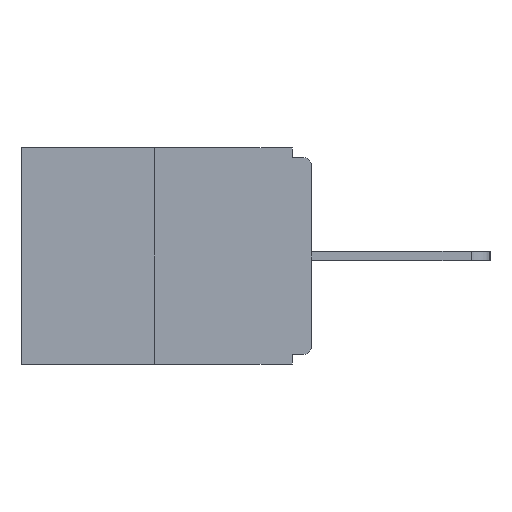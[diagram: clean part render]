
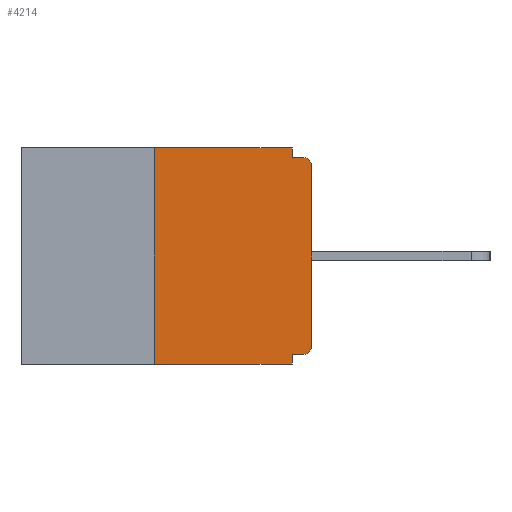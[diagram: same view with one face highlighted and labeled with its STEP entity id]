
A CAD part, left-side view. The second image highlights one B-rep face of the part: STEP entity #4214.
In plain terms, the highlighted planar face has unit normal (-1, 0, 0).
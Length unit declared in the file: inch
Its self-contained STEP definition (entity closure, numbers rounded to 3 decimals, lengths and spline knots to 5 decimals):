
#323 = AXIS2_PLACEMENT_3D ( 'NONE', #721, #25319, #17155 ) ;
#538 = ORIENTED_EDGE ( 'NONE', *, *, #24156, .F. ) ;
#721 = CARTESIAN_POINT ( 'NONE',  ( 0., 0.46, 0. ) ) ;
#915 = VECTOR ( 'NONE', #14910, 39.37008 ) ;
#925 = ORIENTED_EDGE ( 'NONE', *, *, #1506, .F. ) ;
#1203 = DIRECTION ( 'NONE',  ( 0., 0., -1. ) ) ;
#1506 = EDGE_CURVE ( 'NONE', #7267, #21298, #11425, .T. ) ;
#1704 = AXIS2_PLACEMENT_3D ( 'NONE', #9075, #2961, #7179 ) ;
#1990 = CARTESIAN_POINT ( 'NONE',  ( 0., 0.031, -0.015 ) ) ;
#2344 = EDGE_CURVE ( 'NONE', #15283, #7643, #25495, .T. ) ;
#2492 = FACE_OUTER_BOUND ( 'NONE', #23433, .T. ) ;
#2899 = EDGE_CURVE ( 'NONE', #25150, #3017, #26515, .T. ) ;
#2961 = DIRECTION ( 'NONE',  ( -1., 0., 0. ) ) ;
#3017 = VERTEX_POINT ( 'NONE', #17044 ) ;
#3369 = ORIENTED_EDGE ( 'NONE', *, *, #12321, .T. ) ;
#4214 = ADVANCED_FACE ( 'NONE', ( #2492 ), #15115, .F. ) ;
#4600 = CARTESIAN_POINT ( 'NONE',  ( 0., 0.25, -0.343 ) ) ;
#4879 = ORIENTED_EDGE ( 'NONE', *, *, #2899, .F. ) ;
#5553 = ORIENTED_EDGE ( 'NONE', *, *, #2344, .T. ) ;
#6460 = CIRCLE ( 'NONE', #22078, 0.015 ) ;
#6619 = CARTESIAN_POINT ( 'NONE',  ( 0., 0., -0.015 ) ) ;
#6686 = VECTOR ( 'NONE', #24481, 39.37008 ) ;
#6695 = ORIENTED_EDGE ( 'NONE', *, *, #18225, .F. ) ;
#6821 = LINE ( 'NONE', #12928, #9926 ) ;
#7179 = DIRECTION ( 'NONE',  ( 0., 0., -1. ) ) ;
#7267 = VERTEX_POINT ( 'NONE', #20975 ) ;
#7643 = VERTEX_POINT ( 'NONE', #8574 ) ;
#8574 = CARTESIAN_POINT ( 'NONE',  ( 0., 0., -0.03 ) ) ;
#9075 = CARTESIAN_POINT ( 'NONE',  ( 0., 0.015, -0.03 ) ) ;
#9462 = CARTESIAN_POINT ( 'NONE',  ( 0., 0., 0. ) ) ;
#9488 = CARTESIAN_POINT ( 'NONE',  ( 0., 0.031, 0. ) ) ;
#9853 = VECTOR ( 'NONE', #26040, 39.37008 ) ;
#9926 = VECTOR ( 'NONE', #13343, 39.37008 ) ;
#10602 = VERTEX_POINT ( 'NONE', #1990 ) ;
#10863 = CARTESIAN_POINT ( 'NONE',  ( 0., 0., -0.313 ) ) ;
#11134 = LINE ( 'NONE', #20710, #16124 ) ;
#11425 = LINE ( 'NONE', #15916, #22614 ) ;
#11450 = EDGE_CURVE ( 'NONE', #25150, #21298, #6821, .T. ) ;
#11519 = CARTESIAN_POINT ( 'NONE',  ( 0., 0.015, -0.313 ) ) ;
#12146 = CARTESIAN_POINT ( 'NONE',  ( 0., 0.031, -0.343 ) ) ;
#12321 = EDGE_CURVE ( 'NONE', #7643, #13069, #25129, .T. ) ;
#12851 = CARTESIAN_POINT ( 'NONE',  ( 0., 0.015, -0.328 ) ) ;
#12928 = CARTESIAN_POINT ( 'NONE',  ( 0., 0.46, -0.343 ) ) ;
#13044 = VECTOR ( 'NONE', #1203, 39.37008 ) ;
#13069 = VERTEX_POINT ( 'NONE', #13161 ) ;
#13161 = CARTESIAN_POINT ( 'NONE',  ( 0., 0.015, -0.015 ) ) ;
#13243 = CARTESIAN_POINT ( 'NONE',  ( 0., 0., -0.328 ) ) ;
#13343 = DIRECTION ( 'NONE',  ( 0., -1., 0. ) ) ;
#14123 = DIRECTION ( 'NONE',  ( -1., 0., 0. ) ) ;
#14910 = DIRECTION ( 'NONE',  ( 0., -1., 0. ) ) ;
#15115 = PLANE ( 'NONE',  #323 ) ;
#15283 = VERTEX_POINT ( 'NONE', #10863 ) ;
#15684 = ORIENTED_EDGE ( 'NONE', *, *, #26019, .F. ) ;
#15788 = DIRECTION ( 'NONE',  ( 0., 0., -1. ) ) ;
#15916 = CARTESIAN_POINT ( 'NONE',  ( 0., 0.031, -0.343 ) ) ;
#16124 = VECTOR ( 'NONE', #24782, 39.37008 ) ;
#16198 = CARTESIAN_POINT ( 'NONE',  ( 0., 0.25, 0. ) ) ;
#17044 = CARTESIAN_POINT ( 'NONE',  ( 0., 0.25, 0. ) ) ;
#17155 = DIRECTION ( 'NONE',  ( 0., 0., -1. ) ) ;
#18225 = EDGE_CURVE ( 'NONE', #24071, #7267, #25875, .T. ) ;
#18526 = ORIENTED_EDGE ( 'NONE', *, *, #22008, .T. ) ;
#18573 = VERTEX_POINT ( 'NONE', #19194 ) ;
#19194 = CARTESIAN_POINT ( 'NONE',  ( 0., 0.031, 0. ) ) ;
#19361 = DIRECTION ( 'NONE',  ( 0., 1., 0. ) ) ;
#20710 = CARTESIAN_POINT ( 'NONE',  ( 0., 0.46, 0. ) ) ;
#20907 = VECTOR ( 'NONE', #19361, 39.37008 ) ;
#20975 = CARTESIAN_POINT ( 'NONE',  ( 0., 0.031, -0.328 ) ) ;
#21298 = VERTEX_POINT ( 'NONE', #12146 ) ;
#22008 = EDGE_CURVE ( 'NONE', #24071, #15283, #6460, .T. ) ;
#22078 = AXIS2_PLACEMENT_3D ( 'NONE', #11519, #14123, #24043 ) ;
#22112 = LINE ( 'NONE', #9488, #13044 ) ;
#22132 = ORIENTED_EDGE ( 'NONE', *, *, #23838, .F. ) ;
#22163 = ORIENTED_EDGE ( 'NONE', *, *, #11450, .T. ) ;
#22614 = VECTOR ( 'NONE', #15788, 39.37008 ) ;
#23433 = EDGE_LOOP ( 'NONE', ( #15684, #4879, #22163, #925, #6695, #18526, #5553, #3369, #538, #22132 ) ) ;
#23838 = EDGE_CURVE ( 'NONE', #18573, #10602, #22112, .T. ) ;
#24043 = DIRECTION ( 'NONE',  ( 0., 0., -1. ) ) ;
#24071 = VERTEX_POINT ( 'NONE', #12851 ) ;
#24156 = EDGE_CURVE ( 'NONE', #10602, #13069, #25228, .T. ) ;
#24481 = DIRECTION ( 'NONE',  ( 0., 0., 1. ) ) ;
#24782 = DIRECTION ( 'NONE',  ( 0., -1., 0. ) ) ;
#25129 = CIRCLE ( 'NONE', #1704, 0.015 ) ;
#25150 = VERTEX_POINT ( 'NONE', #4600 ) ;
#25228 = LINE ( 'NONE', #6619, #915 ) ;
#25319 = DIRECTION ( 'NONE',  ( 1., 0., 0. ) ) ;
#25495 = LINE ( 'NONE', #9462, #9853 ) ;
#25875 = LINE ( 'NONE', #13243, #20907 ) ;
#26019 = EDGE_CURVE ( 'NONE', #3017, #18573, #11134, .T. ) ;
#26040 = DIRECTION ( 'NONE',  ( 0., 0., 1. ) ) ;
#26515 = LINE ( 'NONE', #16198, #6686 ) ;
